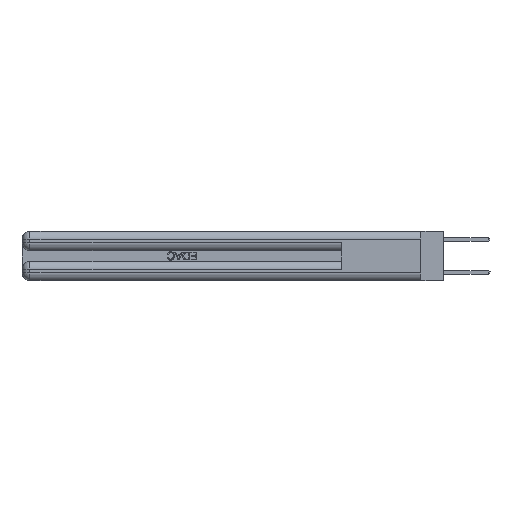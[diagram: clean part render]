
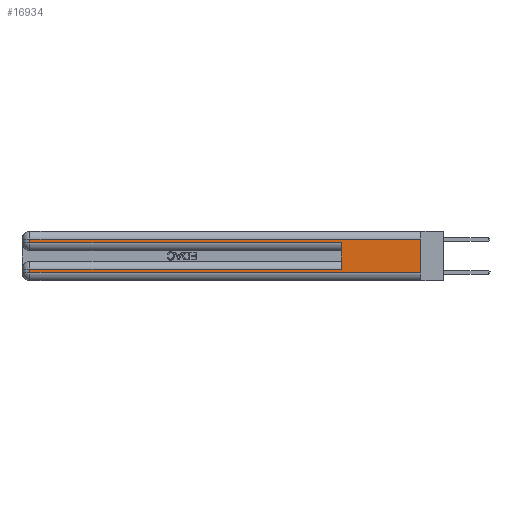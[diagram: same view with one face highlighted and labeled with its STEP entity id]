
A CAD part, left-side view. The second image highlights one B-rep face of the part: STEP entity #16934.
In plain terms, the highlighted planar face has unit normal (-1, 0, 0).
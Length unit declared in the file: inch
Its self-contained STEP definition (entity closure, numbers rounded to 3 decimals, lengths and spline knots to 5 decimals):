
#34 = ORIENTED_EDGE ( 'NONE', *, *, #16256, .T. ) ;
#363 = CARTESIAN_POINT ( 'NONE',  ( 0., 0., 0.285 ) ) ;
#456 = ORIENTED_EDGE ( 'NONE', *, *, #5217, .T. ) ;
#1140 = VECTOR ( 'NONE', #26573, 39.37008 ) ;
#1234 = EDGE_LOOP ( 'NONE', ( #10543, #21627, #34, #27143, #22934, #23890, #10547, #456 ) ) ;
#2636 = VECTOR ( 'NONE', #9700, 39.37008 ) ;
#2912 = FACE_OUTER_BOUND ( 'NONE', #1234, .T. ) ;
#4862 = CARTESIAN_POINT ( 'NONE',  ( 0., 0., 0.085 ) ) ;
#5217 = EDGE_CURVE ( 'NONE', #5670, #17335, #14019, .T. ) ;
#5269 = CARTESIAN_POINT ( 'NONE',  ( 0., 2.94, 0.06 ) ) ;
#5528 = CARTESIAN_POINT ( 'NONE',  ( 0., 0.6, 0.285 ) ) ;
#5670 = VERTEX_POINT ( 'NONE', #5269 ) ;
#5938 = DIRECTION ( 'NONE',  ( 1., 0., 0. ) ) ;
#7060 = VECTOR ( 'NONE', #17764, 39.37008 ) ;
#7219 = DIRECTION ( 'NONE',  ( 0., 1., 0. ) ) ;
#7338 = LINE ( 'NONE', #12515, #1140 ) ;
#7380 = VERTEX_POINT ( 'NONE', #23790 ) ;
#7396 = VECTOR ( 'NONE', #14926, 39.37008 ) ;
#8499 = VERTEX_POINT ( 'NONE', #8648 ) ;
#8648 = CARTESIAN_POINT ( 'NONE',  ( 0., 0.6, 0.085 ) ) ;
#8755 = CARTESIAN_POINT ( 'NONE',  ( 0., 2.94, 0.285 ) ) ;
#9700 = DIRECTION ( 'NONE',  ( 0., -1., 0. ) ) ;
#10543 = ORIENTED_EDGE ( 'NONE', *, *, #28497, .F. ) ;
#10547 = ORIENTED_EDGE ( 'NONE', *, *, #29594, .T. ) ;
#10947 = VERTEX_POINT ( 'NONE', #8755 ) ;
#11950 = EDGE_CURVE ( 'NONE', #7380, #19735, #29711, .T. ) ;
#12515 = CARTESIAN_POINT ( 'NONE',  ( 0., 2.94, 0.37 ) ) ;
#12595 = CARTESIAN_POINT ( 'NONE',  ( 0., 2.94, 0.37 ) ) ;
#13257 = CARTESIAN_POINT ( 'NONE',  ( 0., 0., 0.37 ) ) ;
#14019 = LINE ( 'NONE', #24683, #7060 ) ;
#14570 = LINE ( 'NONE', #4862, #26241 ) ;
#14926 = DIRECTION ( 'NONE',  ( 0., 0., -1. ) ) ;
#15020 = CARTESIAN_POINT ( 'NONE',  ( 0., 0., 0.31 ) ) ;
#15066 = LINE ( 'NONE', #12595, #7396 ) ;
#15232 = PLANE ( 'NONE',  #15935 ) ;
#15378 = EDGE_CURVE ( 'NONE', #8499, #23018, #23100, .T. ) ;
#15935 = AXIS2_PLACEMENT_3D ( 'NONE', #19924, #5938, #22260 ) ;
#16256 = EDGE_CURVE ( 'NONE', #19735, #10947, #7338, .T. ) ;
#16621 = DIRECTION ( 'NONE',  ( 0., 0., 1. ) ) ;
#16628 = CARTESIAN_POINT ( 'NONE',  ( 0., 0., 0.06 ) ) ;
#16934 = ADVANCED_FACE ( 'NONE', ( #2912 ), #15232, .F. ) ;
#17335 = VERTEX_POINT ( 'NONE', #16628 ) ;
#17764 = DIRECTION ( 'NONE',  ( 0., -1., 0. ) ) ;
#18219 = CARTESIAN_POINT ( 'NONE',  ( 0., 2.94, 0.085 ) ) ;
#19735 = VERTEX_POINT ( 'NONE', #27081 ) ;
#19924 = CARTESIAN_POINT ( 'NONE',  ( 0., 0., 0.37 ) ) ;
#20302 = DIRECTION ( 'NONE',  ( 0., 0., -1. ) ) ;
#21627 = ORIENTED_EDGE ( 'NONE', *, *, #11950, .T. ) ;
#22175 = EDGE_CURVE ( 'NONE', #8499, #26106, #14570, .T. ) ;
#22260 = DIRECTION ( 'NONE',  ( 0., 0., -1. ) ) ;
#22358 = VECTOR ( 'NONE', #16621, 39.37008 ) ;
#22375 = VECTOR ( 'NONE', #20302, 39.37008 ) ;
#22934 = ORIENTED_EDGE ( 'NONE', *, *, #15378, .F. ) ;
#23018 = VERTEX_POINT ( 'NONE', #5528 ) ;
#23100 = LINE ( 'NONE', #28252, #22358 ) ;
#23121 = LINE ( 'NONE', #13257, #22375 ) ;
#23790 = CARTESIAN_POINT ( 'NONE',  ( 0., 0., 0.31 ) ) ;
#23890 = ORIENTED_EDGE ( 'NONE', *, *, #22175, .T. ) ;
#24272 = VECTOR ( 'NONE', #28965, 39.37008 ) ;
#24683 = CARTESIAN_POINT ( 'NONE',  ( 0., 0., 0.06 ) ) ;
#26106 = VERTEX_POINT ( 'NONE', #18219 ) ;
#26241 = VECTOR ( 'NONE', #7219, 39.37008 ) ;
#26573 = DIRECTION ( 'NONE',  ( 0., 0., -1. ) ) ;
#27081 = CARTESIAN_POINT ( 'NONE',  ( 0., 2.94, 0.31 ) ) ;
#27143 = ORIENTED_EDGE ( 'NONE', *, *, #28808, .T. ) ;
#28252 = CARTESIAN_POINT ( 'NONE',  ( 0., 0.6, 0.145 ) ) ;
#28497 = EDGE_CURVE ( 'NONE', #7380, #17335, #23121, .T. ) ;
#28808 = EDGE_CURVE ( 'NONE', #10947, #23018, #28912, .T. ) ;
#28912 = LINE ( 'NONE', #363, #2636 ) ;
#28965 = DIRECTION ( 'NONE',  ( 0., 1., 0. ) ) ;
#29594 = EDGE_CURVE ( 'NONE', #26106, #5670, #15066, .T. ) ;
#29711 = LINE ( 'NONE', #15020, #24272 ) ;
